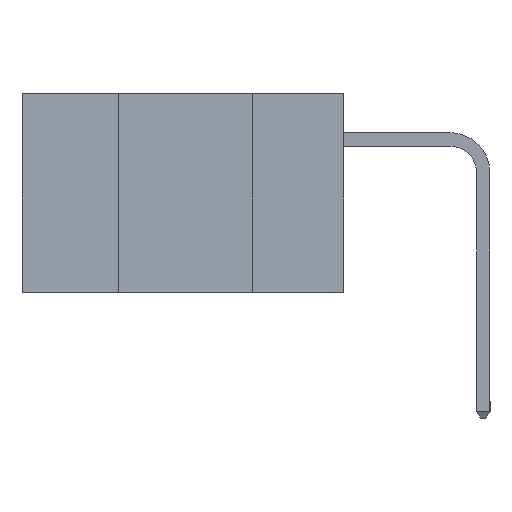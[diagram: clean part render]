
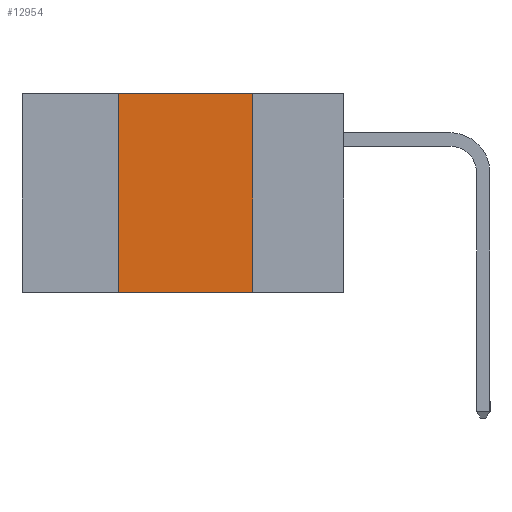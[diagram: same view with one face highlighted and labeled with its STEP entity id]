
A CAD part, left-side view. The second image highlights one B-rep face of the part: STEP entity #12954.
In plain terms, the highlighted planar face has unit normal (-1, 0, 0).
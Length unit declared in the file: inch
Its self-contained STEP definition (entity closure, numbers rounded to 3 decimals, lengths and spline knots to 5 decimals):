
#7 = ORIENTED_EDGE ( 'NONE', *, *, #5025, .F. ) ;
#156 = CARTESIAN_POINT ( 'NONE',  ( 0., 0.42, 0. ) ) ;
#159 = CARTESIAN_POINT ( 'NONE',  ( 0., 0.6, 0. ) ) ;
#336 = DIRECTION ( 'NONE',  ( 0., -1., 0. ) ) ;
#551 = VECTOR ( 'NONE', #18313, 39.37008 ) ;
#1283 = CARTESIAN_POINT ( 'NONE',  ( 0., 0.17, 0. ) ) ;
#2581 = ORIENTED_EDGE ( 'NONE', *, *, #13693, .T. ) ;
#3225 = LINE ( 'NONE', #17176, #7177 ) ;
#3269 = CARTESIAN_POINT ( 'NONE',  ( 0., 0.6, -0.37 ) ) ;
#4152 = CARTESIAN_POINT ( 'NONE',  ( 0., 0.17, -0.37 ) ) ;
#4968 = VERTEX_POINT ( 'NONE', #13332 ) ;
#5025 = EDGE_CURVE ( 'NONE', #4968, #12937, #7461, .T. ) ;
#7177 = VECTOR ( 'NONE', #18521, 39.37008 ) ;
#7461 = LINE ( 'NONE', #18567, #11788 ) ;
#7636 = CARTESIAN_POINT ( 'NONE',  ( 0., 0.6, 0. ) ) ;
#7722 = AXIS2_PLACEMENT_3D ( 'NONE', #7636, #17577, #9114 ) ;
#7863 = EDGE_CURVE ( 'NONE', #12937, #10719, #8457, .T. ) ;
#7923 = VECTOR ( 'NONE', #336, 39.37008 ) ;
#8457 = LINE ( 'NONE', #159, #551 ) ;
#9101 = FACE_OUTER_BOUND ( 'NONE', #14505, .T. ) ;
#9114 = DIRECTION ( 'NONE',  ( 0., 0., -1. ) ) ;
#10522 = PLANE ( 'NONE',  #7722 ) ;
#10710 = EDGE_CURVE ( 'NONE', #10719, #12845, #3225, .T. ) ;
#10719 = VERTEX_POINT ( 'NONE', #1283 ) ;
#11788 = VECTOR ( 'NONE', #18499, 39.37008 ) ;
#11791 = LINE ( 'NONE', #3269, #7923 ) ;
#12845 = VERTEX_POINT ( 'NONE', #4152 ) ;
#12937 = VERTEX_POINT ( 'NONE', #156 ) ;
#12954 = ADVANCED_FACE ( 'NONE', ( #9101 ), #10522, .F. ) ;
#13332 = CARTESIAN_POINT ( 'NONE',  ( 0., 0.42, -0.37 ) ) ;
#13693 = EDGE_CURVE ( 'NONE', #4968, #12845, #11791, .T. ) ;
#14234 = ORIENTED_EDGE ( 'NONE', *, *, #7863, .F. ) ;
#14505 = EDGE_LOOP ( 'NONE', ( #18304, #14234, #7, #2581 ) ) ;
#17176 = CARTESIAN_POINT ( 'NONE',  ( 0., 0.17, -0.37 ) ) ;
#17577 = DIRECTION ( 'NONE',  ( 1., 0., 0. ) ) ;
#18304 = ORIENTED_EDGE ( 'NONE', *, *, #10710, .F. ) ;
#18313 = DIRECTION ( 'NONE',  ( 0., -1., 0. ) ) ;
#18499 = DIRECTION ( 'NONE',  ( 0., 0., 1. ) ) ;
#18521 = DIRECTION ( 'NONE',  ( 0., 0., -1. ) ) ;
#18567 = CARTESIAN_POINT ( 'NONE',  ( 0., 0.42, -0.37 ) ) ;
